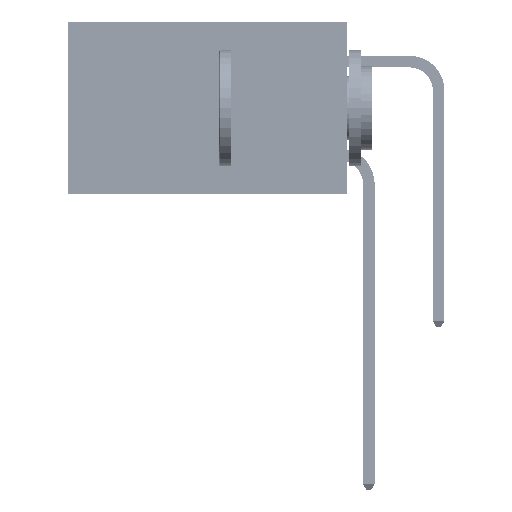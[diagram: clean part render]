
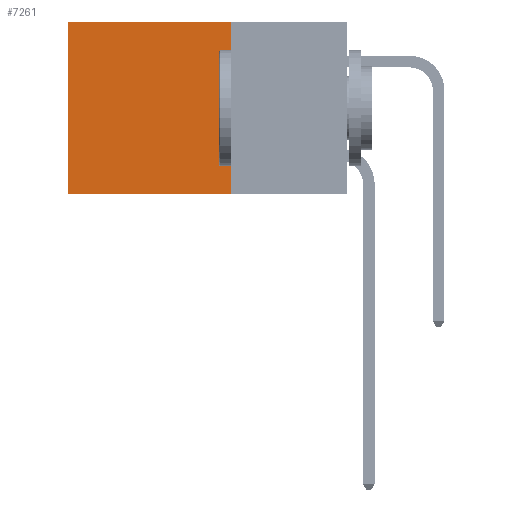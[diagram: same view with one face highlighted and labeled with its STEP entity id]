
A CAD part, left-side view. The second image highlights one B-rep face of the part: STEP entity #7261.
In plain terms, the highlighted planar face has unit normal (-1, 0, 0).
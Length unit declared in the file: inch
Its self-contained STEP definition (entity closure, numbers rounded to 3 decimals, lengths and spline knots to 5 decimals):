
#2198 = ORIENTED_EDGE ( 'NONE', *, *, #20373, .F. ) ;
#2448 = VECTOR ( 'NONE', #22590, 39.37008 ) ;
#2711 = LINE ( 'NONE', #28149, #17851 ) ;
#2778 = PLANE ( 'NONE',  #49052 ) ;
#3195 = VERTEX_POINT ( 'NONE', #30660 ) ;
#4144 = EDGE_CURVE ( 'NONE', #3195, #14589, #14742, .T. ) ;
#4293 = VECTOR ( 'NONE', #22420, 39.37008 ) ;
#5802 = LINE ( 'NONE', #16418, #25467 ) ;
#6221 = ORIENTED_EDGE ( 'NONE', *, *, #4144, .T. ) ;
#6705 = DIRECTION ( 'NONE',  ( 0., 0., -1. ) ) ;
#7261 = ADVANCED_FACE ( 'NONE', ( #24842 ), #2778, .F. ) ;
#13851 = EDGE_LOOP ( 'NONE', ( #16713, #2198, #17670, #6221 ) ) ;
#14589 = VERTEX_POINT ( 'NONE', #36709 ) ;
#14742 = LINE ( 'NONE', #41866, #4293 ) ;
#16418 = CARTESIAN_POINT ( 'NONE',  ( 0.2875, 0.25, 0. ) ) ;
#16713 = ORIENTED_EDGE ( 'NONE', *, *, #36955, .T. ) ;
#17670 = ORIENTED_EDGE ( 'NONE', *, *, #32447, .F. ) ;
#17851 = VECTOR ( 'NONE', #39876, 39.37008 ) ;
#18366 = VERTEX_POINT ( 'NONE', #22993 ) ;
#19697 = VERTEX_POINT ( 'NONE', #24777 ) ;
#20373 = EDGE_CURVE ( 'NONE', #18366, #19697, #2711, .T. ) ;
#22420 = DIRECTION ( 'NONE',  ( 0., 1., 0. ) ) ;
#22590 = DIRECTION ( 'NONE',  ( 0., 0., -1. ) ) ;
#22993 = CARTESIAN_POINT ( 'NONE',  ( 0.2875, 0.25, -0.37 ) ) ;
#24777 = CARTESIAN_POINT ( 'NONE',  ( 0.2875, 0.6, -0.37 ) ) ;
#24842 = FACE_OUTER_BOUND ( 'NONE', #13851, .T. ) ;
#25467 = VECTOR ( 'NONE', #32348, 39.37008 ) ;
#28149 = CARTESIAN_POINT ( 'NONE',  ( 0.2875, 0.25, -0.37 ) ) ;
#30196 = DIRECTION ( 'NONE',  ( 1., 0., 0. ) ) ;
#30660 = CARTESIAN_POINT ( 'NONE',  ( 0.2875, 0.25, 0. ) ) ;
#32348 = DIRECTION ( 'NONE',  ( 0., 0., -1. ) ) ;
#32447 = EDGE_CURVE ( 'NONE', #3195, #18366, #5802, .T. ) ;
#34001 = CARTESIAN_POINT ( 'NONE',  ( 0.2875, 0.25, 0. ) ) ;
#36709 = CARTESIAN_POINT ( 'NONE',  ( 0.2875, 0.6, 0. ) ) ;
#36955 = EDGE_CURVE ( 'NONE', #14589, #19697, #44267, .T. ) ;
#39876 = DIRECTION ( 'NONE',  ( 0., 1., 0. ) ) ;
#41866 = CARTESIAN_POINT ( 'NONE',  ( 0.2875, 0.25, 0. ) ) ;
#44267 = LINE ( 'NONE', #46485, #2448 ) ;
#46485 = CARTESIAN_POINT ( 'NONE',  ( 0.2875, 0.6, 0. ) ) ;
#49052 = AXIS2_PLACEMENT_3D ( 'NONE', #34001, #30196, #6705 ) ;
